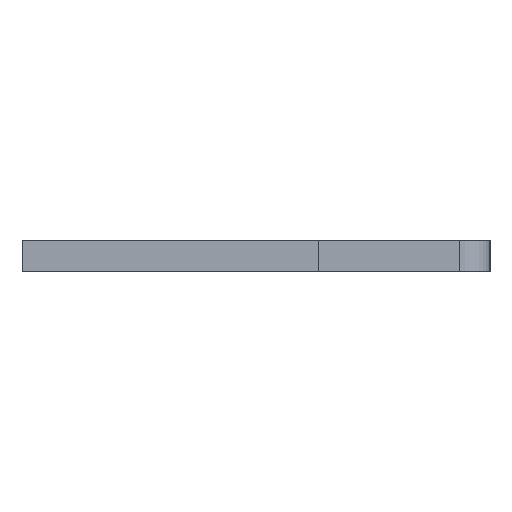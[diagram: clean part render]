
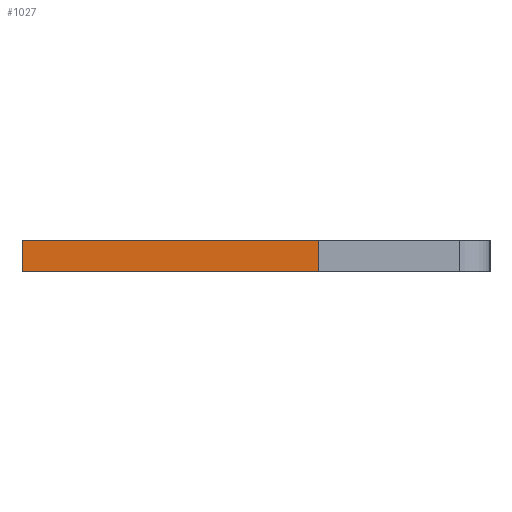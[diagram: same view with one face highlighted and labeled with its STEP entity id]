
A CAD part, left-side view. The second image highlights one B-rep face of the part: STEP entity #1027.
In plain terms, the highlighted face is planar.
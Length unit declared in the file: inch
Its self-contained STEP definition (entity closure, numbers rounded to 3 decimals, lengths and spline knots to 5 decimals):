
#17 = DIRECTION ( 'NONE',  ( -1., 0., 0. ) ) ;
#109 = PLANE ( 'NONE',  #582 ) ;
#122 = VERTEX_POINT ( 'NONE', #1081 ) ;
#160 = DIRECTION ( 'NONE',  ( 0., 1., 0. ) ) ;
#194 = EDGE_CURVE ( 'NONE', #564, #1188, #1478, .T. ) ;
#210 = CARTESIAN_POINT ( 'NONE',  ( 0.01, 0.15, -0.04 ) ) ;
#213 = LINE ( 'NONE', #1353, #477 ) ;
#219 = VECTOR ( 'NONE', #17, 39.37008 ) ;
#250 = DIRECTION ( 'NONE',  ( 0., 0., 1. ) ) ;
#252 = EDGE_CURVE ( 'NONE', #122, #564, #213, .T. ) ;
#259 = DIRECTION ( 'NONE',  ( 1., 0., 0. ) ) ;
#410 = CARTESIAN_POINT ( 'NONE',  ( -0.01, 0.15, -0.04 ) ) ;
#456 = ORIENTED_EDGE ( 'NONE', *, *, #1139, .F. ) ;
#458 = DIRECTION ( 'NONE',  ( 0., 1., 0. ) ) ;
#477 = VECTOR ( 'NONE', #530, 39.37008 ) ;
#480 = LINE ( 'NONE', #716, #219 ) ;
#530 = DIRECTION ( 'NONE',  ( -1., 0., 0. ) ) ;
#564 = VERTEX_POINT ( 'NONE', #678 ) ;
#582 = AXIS2_PLACEMENT_3D ( 'NONE', #706, #250, #259 ) ;
#591 = CARTESIAN_POINT ( 'NONE',  ( -0.01, 0.15, -0.04 ) ) ;
#634 = VERTEX_POINT ( 'NONE', #210 ) ;
#675 = EDGE_LOOP ( 'NONE', ( #1368, #456, #1465, #1360 ) ) ;
#678 = CARTESIAN_POINT ( 'NONE',  ( -0.01, -0.04, -0.04 ) ) ;
#706 = CARTESIAN_POINT ( 'NONE',  ( 0.01, 0.15, -0.04 ) ) ;
#716 = CARTESIAN_POINT ( 'NONE',  ( 0.01, 0.15, -0.04 ) ) ;
#733 = FACE_OUTER_BOUND ( 'NONE', #675, .T. ) ;
#804 = LINE ( 'NONE', #827, #929 ) ;
#827 = CARTESIAN_POINT ( 'NONE',  ( 0.01, 0.15, -0.04 ) ) ;
#929 = VECTOR ( 'NONE', #458, 39.37008 ) ;
#1010 = EDGE_CURVE ( 'NONE', #122, #634, #804, .T. ) ;
#1027 = ADVANCED_FACE ( 'NONE', ( #733 ), #109, .F. ) ;
#1081 = CARTESIAN_POINT ( 'NONE',  ( 0.01, -0.04, -0.04 ) ) ;
#1139 = EDGE_CURVE ( 'NONE', #634, #1188, #480, .T. ) ;
#1173 = VECTOR ( 'NONE', #160, 39.37008 ) ;
#1188 = VERTEX_POINT ( 'NONE', #591 ) ;
#1353 = CARTESIAN_POINT ( 'NONE',  ( 0.01, -0.04, -0.04 ) ) ;
#1360 = ORIENTED_EDGE ( 'NONE', *, *, #252, .T. ) ;
#1368 = ORIENTED_EDGE ( 'NONE', *, *, #194, .T. ) ;
#1465 = ORIENTED_EDGE ( 'NONE', *, *, #1010, .F. ) ;
#1478 = LINE ( 'NONE', #410, #1173 ) ;
